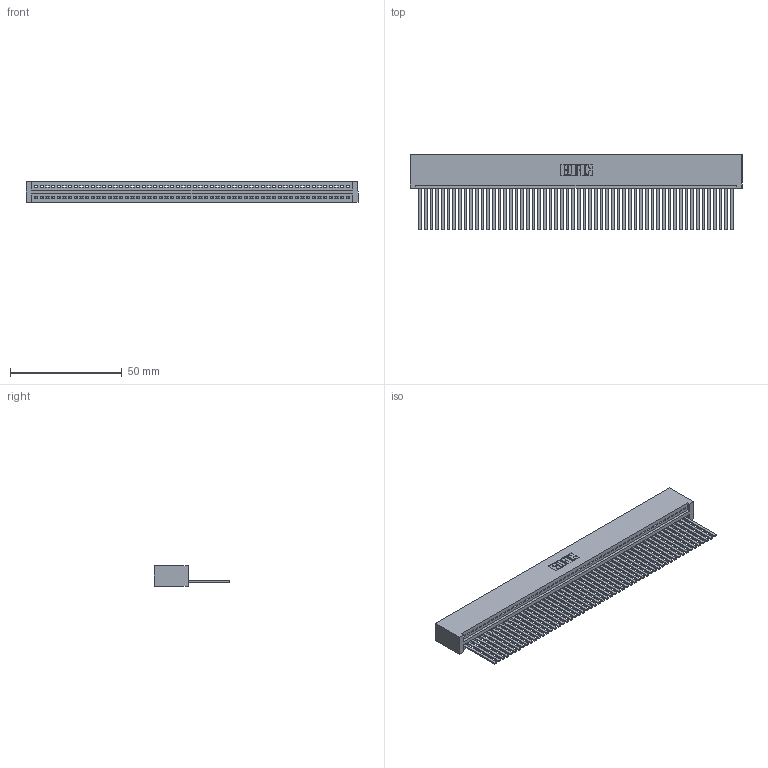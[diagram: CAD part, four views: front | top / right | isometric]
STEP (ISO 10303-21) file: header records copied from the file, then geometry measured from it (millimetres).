
FILE_DESCRIPTION (( 'STEP AP203' ), '1' );
FILE_NAME ('345-056-544-101.STEP', '2019-10-10T11:45:18', ( '' ), ( '' ), 'SwSTEP 2.0', 'SolidWorks 2016', '' );
FILE_SCHEMA (( 'CONFIG_CONTROL_DESIGN' ));
Length unit declared in the file: inch
Products named in the file (3): 345-292-001_345-293-144; 345 Part_No Mounting Lugs; 345-056-544-101
Assembly tree (57 placements, depth 2):
  345-056-544-101
    345 Part_No Mounting Lugs
    345-292-001_345-293-144  x56
Bounding box: 148.84 x 33.96 x 9.4 mm (x, y, z)
Volume: 15484.9 mm3; surface area: 22905.5 mm2
Topology: 57 solids, 57 shells, 3030 faces, 9165 edges, 6034 vertices
Faces by surface type: plane 2092, cylinder 938
Entity records: 39801 total; most frequent: CARTESIAN_POINT 6900, ORIENTED_EDGE 6890, DIRECTION 5997, EDGE_CURVE 3445, LINE 3101, VECTOR 3101, VERTEX_POINT 2294, AXIS2_PLACEMENT_3D 1448
